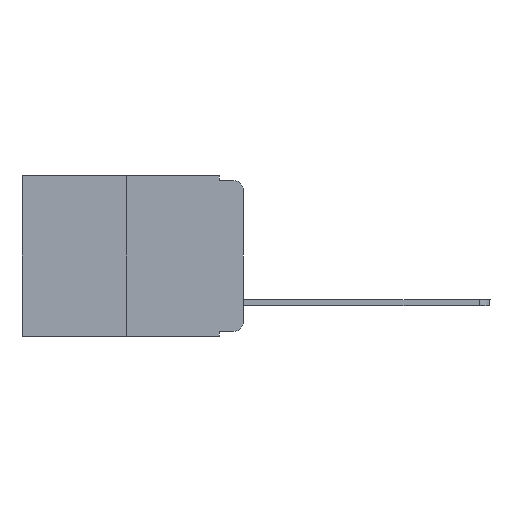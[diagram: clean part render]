
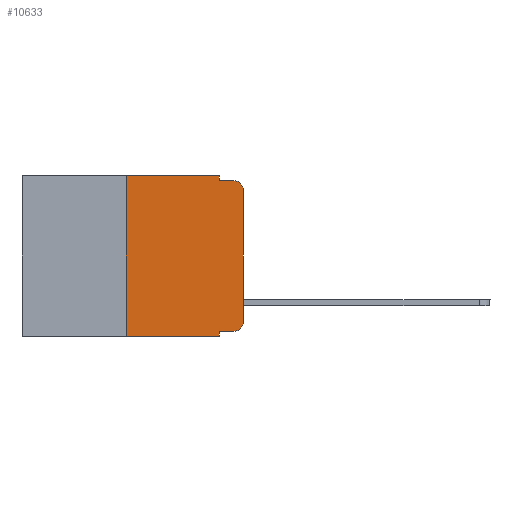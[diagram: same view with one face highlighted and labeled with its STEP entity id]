
A CAD part, left-side view. The second image highlights one B-rep face of the part: STEP entity #10633.
In plain terms, the highlighted planar face has unit normal (-1, 0, 0).
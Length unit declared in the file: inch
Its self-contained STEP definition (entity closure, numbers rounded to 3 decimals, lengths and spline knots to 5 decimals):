
#90 = VERTEX_POINT ( 'NONE', #15511 ) ;
#268 = VECTOR ( 'NONE', #20372, 39.37008 ) ;
#873 = VECTOR ( 'NONE', #13523, 39.37008 ) ;
#1294 = AXIS2_PLACEMENT_3D ( 'NONE', #17371, #7881, #18999 ) ;
#1317 = CIRCLE ( 'NONE', #6314, 0.02 ) ;
#1580 = EDGE_CURVE ( 'NONE', #7033, #7132, #17335, .T. ) ;
#1809 = ORIENTED_EDGE ( 'NONE', *, *, #2090, .T. ) ;
#2090 = EDGE_CURVE ( 'NONE', #5577, #90, #19307, .T. ) ;
#2276 = CARTESIAN_POINT ( 'NONE',  ( 0., 0.02, -0.03 ) ) ;
#3028 = DIRECTION ( 'NONE',  ( 0., -1., 0. ) ) ;
#3305 = VERTEX_POINT ( 'NONE', #3857 ) ;
#3470 = CARTESIAN_POINT ( 'NONE',  ( 0., 0.02, -0.01 ) ) ;
#3857 = CARTESIAN_POINT ( 'NONE',  ( 0., 0.051, -0.343 ) ) ;
#3877 = EDGE_CURVE ( 'NONE', #8279, #16726, #17238, .T. ) ;
#3888 = CARTESIAN_POINT ( 'NONE',  ( 0., 0.25, 0. ) ) ;
#4361 = AXIS2_PLACEMENT_3D ( 'NONE', #10790, #6210, #18673 ) ;
#4676 = PLANE ( 'NONE',  #1294 ) ;
#4714 = VERTEX_POINT ( 'NONE', #10160 ) ;
#4889 = CARTESIAN_POINT ( 'NONE',  ( 0., 0., 0. ) ) ;
#5122 = ORIENTED_EDGE ( 'NONE', *, *, #11274, .T. ) ;
#5577 = VERTEX_POINT ( 'NONE', #20134 ) ;
#6210 = DIRECTION ( 'NONE',  ( -1., 0., 0. ) ) ;
#6297 = CARTESIAN_POINT ( 'NONE',  ( 0., 0.051, -0.333 ) ) ;
#6314 = AXIS2_PLACEMENT_3D ( 'NONE', #2276, #11725, #14914 ) ;
#6321 = ORIENTED_EDGE ( 'NONE', *, *, #14514, .F. ) ;
#6447 = LINE ( 'NONE', #13595, #18903 ) ;
#7033 = VERTEX_POINT ( 'NONE', #19054 ) ;
#7132 = VERTEX_POINT ( 'NONE', #3470 ) ;
#7775 = CARTESIAN_POINT ( 'NONE',  ( 0., 0.473, -0.343 ) ) ;
#7881 = DIRECTION ( 'NONE',  ( 1., 0., 0. ) ) ;
#7944 = LINE ( 'NONE', #7775, #18374 ) ;
#8279 = VERTEX_POINT ( 'NONE', #11367 ) ;
#8356 = EDGE_CURVE ( 'NONE', #90, #7132, #1317, .T. ) ;
#8848 = CARTESIAN_POINT ( 'NONE',  ( 0., 0.051, 0. ) ) ;
#8895 = VECTOR ( 'NONE', #17387, 39.37008 ) ;
#9137 = ORIENTED_EDGE ( 'NONE', *, *, #15663, .T. ) ;
#9514 = CARTESIAN_POINT ( 'NONE',  ( 0., 0.051, -0.01 ) ) ;
#10160 = CARTESIAN_POINT ( 'NONE',  ( 0., 0.02, -0.333 ) ) ;
#10568 = CIRCLE ( 'NONE', #4361, 0.02 ) ;
#10633 = ADVANCED_FACE ( 'NONE', ( #16316 ), #4676, .F. ) ;
#10790 = CARTESIAN_POINT ( 'NONE',  ( 0., 0.02, -0.313 ) ) ;
#11223 = ORIENTED_EDGE ( 'NONE', *, *, #3877, .F. ) ;
#11274 = EDGE_CURVE ( 'NONE', #15717, #4714, #16036, .T. ) ;
#11367 = CARTESIAN_POINT ( 'NONE',  ( 0., 0.25, 0. ) ) ;
#11725 = DIRECTION ( 'NONE',  ( -1., 0., 0. ) ) ;
#11882 = EDGE_CURVE ( 'NONE', #4714, #5577, #10568, .T. ) ;
#12135 = ORIENTED_EDGE ( 'NONE', *, *, #1580, .F. ) ;
#13226 = ORIENTED_EDGE ( 'NONE', *, *, #8356, .T. ) ;
#13428 = VECTOR ( 'NONE', #19887, 39.37008 ) ;
#13523 = DIRECTION ( 'NONE',  ( 0., -1., 0. ) ) ;
#13595 = CARTESIAN_POINT ( 'NONE',  ( 0., 0.051, 0. ) ) ;
#13757 = EDGE_LOOP ( 'NONE', ( #1809, #13226, #12135, #6321, #11223, #14695, #9137, #17689, #5122, #13917 ) ) ;
#13917 = ORIENTED_EDGE ( 'NONE', *, *, #11882, .T. ) ;
#14270 = EDGE_CURVE ( 'NONE', #14945, #8279, #16632, .T. ) ;
#14514 = EDGE_CURVE ( 'NONE', #16726, #7033, #19387, .T. ) ;
#14695 = ORIENTED_EDGE ( 'NONE', *, *, #14270, .F. ) ;
#14914 = DIRECTION ( 'NONE',  ( 0., 0., -1. ) ) ;
#14945 = VERTEX_POINT ( 'NONE', #18350 ) ;
#15043 = DIRECTION ( 'NONE',  ( 0., 0., -1. ) ) ;
#15252 = CARTESIAN_POINT ( 'NONE',  ( 0., 0.051, -0.333 ) ) ;
#15420 = EDGE_CURVE ( 'NONE', #15717, #3305, #6447, .T. ) ;
#15511 = CARTESIAN_POINT ( 'NONE',  ( 0., 0., -0.03 ) ) ;
#15663 = EDGE_CURVE ( 'NONE', #14945, #3305, #7944, .T. ) ;
#15717 = VERTEX_POINT ( 'NONE', #6297 ) ;
#15749 = VECTOR ( 'NONE', #19231, 39.37008 ) ;
#16036 = LINE ( 'NONE', #15252, #873 ) ;
#16316 = FACE_OUTER_BOUND ( 'NONE', #13757, .T. ) ;
#16347 = CARTESIAN_POINT ( 'NONE',  ( 0., 0.473, 0. ) ) ;
#16632 = LINE ( 'NONE', #3888, #13428 ) ;
#16726 = VERTEX_POINT ( 'NONE', #8848 ) ;
#17086 = VECTOR ( 'NONE', #20343, 39.37008 ) ;
#17238 = LINE ( 'NONE', #16347, #15749 ) ;
#17335 = LINE ( 'NONE', #9514, #17086 ) ;
#17371 = CARTESIAN_POINT ( 'NONE',  ( 0., 0.473, 0. ) ) ;
#17387 = DIRECTION ( 'NONE',  ( 0., 0., 1. ) ) ;
#17689 = ORIENTED_EDGE ( 'NONE', *, *, #15420, .F. ) ;
#18350 = CARTESIAN_POINT ( 'NONE',  ( 0., 0.25, -0.343 ) ) ;
#18374 = VECTOR ( 'NONE', #3028, 39.37008 ) ;
#18673 = DIRECTION ( 'NONE',  ( 0., 0., -1. ) ) ;
#18797 = CARTESIAN_POINT ( 'NONE',  ( 0., 0.051, 0. ) ) ;
#18903 = VECTOR ( 'NONE', #15043, 39.37008 ) ;
#18999 = DIRECTION ( 'NONE',  ( 0., 0., -1. ) ) ;
#19054 = CARTESIAN_POINT ( 'NONE',  ( 0., 0.051, -0.01 ) ) ;
#19231 = DIRECTION ( 'NONE',  ( 0., -1., 0. ) ) ;
#19307 = LINE ( 'NONE', #4889, #8895 ) ;
#19387 = LINE ( 'NONE', #18797, #268 ) ;
#19887 = DIRECTION ( 'NONE',  ( 0., 0., 1. ) ) ;
#20134 = CARTESIAN_POINT ( 'NONE',  ( 0., 0., -0.313 ) ) ;
#20343 = DIRECTION ( 'NONE',  ( 0., -1., 0. ) ) ;
#20372 = DIRECTION ( 'NONE',  ( 0., 0., -1. ) ) ;
